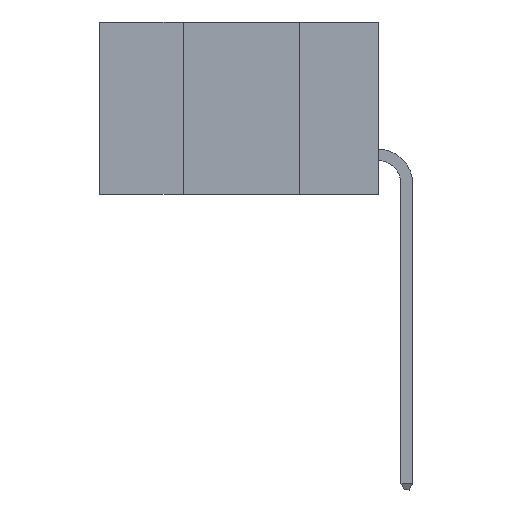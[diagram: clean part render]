
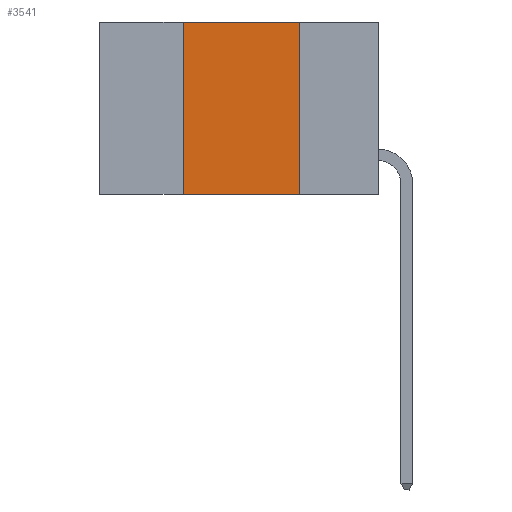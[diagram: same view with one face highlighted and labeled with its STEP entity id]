
A CAD part, left-side view. The second image highlights one B-rep face of the part: STEP entity #3541.
In plain terms, the highlighted planar face has unit normal (-1, 0, 0).
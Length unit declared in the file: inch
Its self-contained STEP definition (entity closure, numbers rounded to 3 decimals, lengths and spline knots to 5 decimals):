
#78 = DIRECTION ( 'NONE',  ( 0., 0., -1. ) ) ;
#729 = VERTEX_POINT ( 'NONE', #12405 ) ;
#790 = LINE ( 'NONE', #3447, #5278 ) ;
#1559 = DIRECTION ( 'NONE',  ( 0., -1., 0. ) ) ;
#1957 = VECTOR ( 'NONE', #5812, 39.37008 ) ;
#2009 = VECTOR ( 'NONE', #1559, 39.37008 ) ;
#2090 = EDGE_LOOP ( 'NONE', ( #5623, #5429, #6285, #6066 ) ) ;
#2724 = VERTEX_POINT ( 'NONE', #8146 ) ;
#3172 = LINE ( 'NONE', #7821, #8071 ) ;
#3447 = CARTESIAN_POINT ( 'NONE',  ( 0., 0.17, 0. ) ) ;
#3541 = ADVANCED_FACE ( 'NONE', ( #9485 ), #5224, .F. ) ;
#3956 = EDGE_CURVE ( 'NONE', #729, #4564, #8210, .T. ) ;
#4564 = VERTEX_POINT ( 'NONE', #10021 ) ;
#4623 = AXIS2_PLACEMENT_3D ( 'NONE', #4791, #5380, #78 ) ;
#4755 = EDGE_CURVE ( 'NONE', #2724, #5316, #3172, .T. ) ;
#4791 = CARTESIAN_POINT ( 'NONE',  ( 0., 0.6, 0. ) ) ;
#5224 = PLANE ( 'NONE',  #4623 ) ;
#5278 = VECTOR ( 'NONE', #11856, 39.37008 ) ;
#5316 = VERTEX_POINT ( 'NONE', #7790 ) ;
#5380 = DIRECTION ( 'NONE',  ( 1., 0., 0. ) ) ;
#5429 = ORIENTED_EDGE ( 'NONE', *, *, #4755, .F. ) ;
#5623 = ORIENTED_EDGE ( 'NONE', *, *, #8481, .F. ) ;
#5812 = DIRECTION ( 'NONE',  ( 0., 0., 1. ) ) ;
#6066 = ORIENTED_EDGE ( 'NONE', *, *, #3956, .T. ) ;
#6285 = ORIENTED_EDGE ( 'NONE', *, *, #6625, .F. ) ;
#6625 = EDGE_CURVE ( 'NONE', #729, #2724, #11767, .T. ) ;
#7790 = CARTESIAN_POINT ( 'NONE',  ( 0., 0.17, 0. ) ) ;
#7821 = CARTESIAN_POINT ( 'NONE',  ( 0., 0.6, 0. ) ) ;
#7825 = DIRECTION ( 'NONE',  ( 0., -1., 0. ) ) ;
#8071 = VECTOR ( 'NONE', #7825, 39.37008 ) ;
#8146 = CARTESIAN_POINT ( 'NONE',  ( 0., 0.42, 0. ) ) ;
#8210 = LINE ( 'NONE', #11774, #2009 ) ;
#8481 = EDGE_CURVE ( 'NONE', #5316, #4564, #790, .T. ) ;
#8900 = CARTESIAN_POINT ( 'NONE',  ( 0., 0.42, 0. ) ) ;
#9485 = FACE_OUTER_BOUND ( 'NONE', #2090, .T. ) ;
#10021 = CARTESIAN_POINT ( 'NONE',  ( 0., 0.17, -0.37 ) ) ;
#11767 = LINE ( 'NONE', #8900, #1957 ) ;
#11774 = CARTESIAN_POINT ( 'NONE',  ( 0., 0.6, -0.37 ) ) ;
#11856 = DIRECTION ( 'NONE',  ( 0., 0., -1. ) ) ;
#12405 = CARTESIAN_POINT ( 'NONE',  ( 0., 0.42, -0.37 ) ) ;
